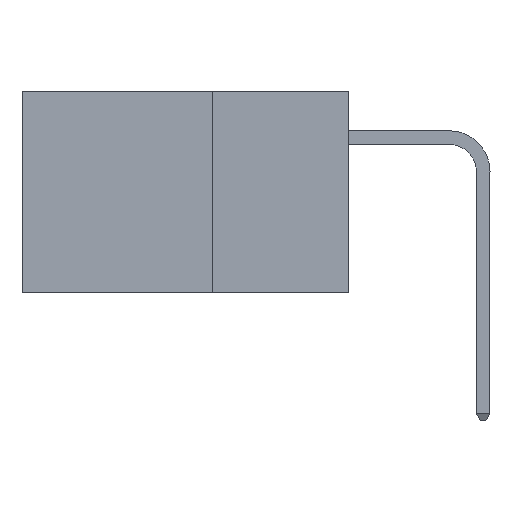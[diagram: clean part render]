
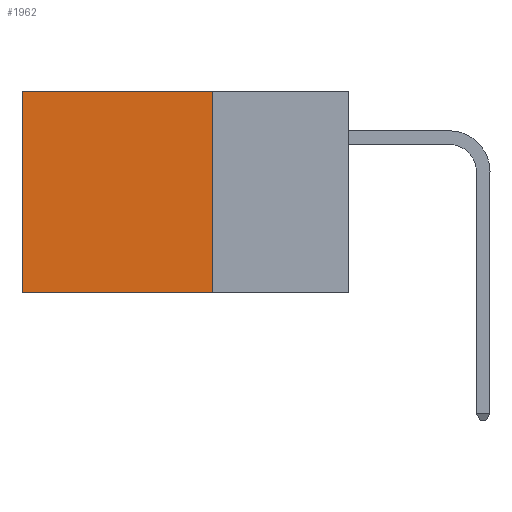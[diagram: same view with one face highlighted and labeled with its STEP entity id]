
A CAD part, left-side view. The second image highlights one B-rep face of the part: STEP entity #1962.
In plain terms, the highlighted planar face has unit normal (-1, 0, 0).
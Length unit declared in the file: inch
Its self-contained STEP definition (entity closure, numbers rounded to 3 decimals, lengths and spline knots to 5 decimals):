
#24 = CARTESIAN_POINT ( 'NONE',  ( 0.2875, 0.25, 0. ) ) ;
#293 = DIRECTION ( 'NONE',  ( 1., 0., 0. ) ) ;
#1059 = LINE ( 'NONE', #8165, #19198 ) ;
#1251 = EDGE_CURVE ( 'NONE', #1690, #9260, #20037, .T. ) ;
#1690 = VERTEX_POINT ( 'NONE', #2579 ) ;
#1962 = ADVANCED_FACE ( 'NONE', ( #7868 ), #17013, .F. ) ;
#2579 = CARTESIAN_POINT ( 'NONE',  ( 0.2875, 0.6, 0. ) ) ;
#2707 = LINE ( 'NONE', #24, #11106 ) ;
#3707 = CARTESIAN_POINT ( 'NONE',  ( 0.2875, 0.25, 0. ) ) ;
#4359 = CARTESIAN_POINT ( 'NONE',  ( 0.2875, 0.25, 0. ) ) ;
#4693 = AXIS2_PLACEMENT_3D ( 'NONE', #3707, #293, #10181 ) ;
#5417 = EDGE_LOOP ( 'NONE', ( #8640, #18408, #6620, #10983 ) ) ;
#6459 = DIRECTION ( 'NONE',  ( 0., 1., 0. ) ) ;
#6620 = ORIENTED_EDGE ( 'NONE', *, *, #13520, .F. ) ;
#6796 = DIRECTION ( 'NONE',  ( 0., 0., -1. ) ) ;
#7310 = VECTOR ( 'NONE', #19511, 39.37008 ) ;
#7457 = CARTESIAN_POINT ( 'NONE',  ( 0.2875, 0.25, 0. ) ) ;
#7610 = CARTESIAN_POINT ( 'NONE',  ( 0.2875, 0.6, 0. ) ) ;
#7868 = FACE_OUTER_BOUND ( 'NONE', #5417, .T. ) ;
#8165 = CARTESIAN_POINT ( 'NONE',  ( 0.2875, 0.25, -0.37 ) ) ;
#8640 = ORIENTED_EDGE ( 'NONE', *, *, #1251, .T. ) ;
#9008 = DIRECTION ( 'NONE',  ( 0., 0., -1. ) ) ;
#9260 = VERTEX_POINT ( 'NONE', #16653 ) ;
#10181 = DIRECTION ( 'NONE',  ( 0., 0., -1. ) ) ;
#10549 = VECTOR ( 'NONE', #9008, 39.37008 ) ;
#10983 = ORIENTED_EDGE ( 'NONE', *, *, #16628, .T. ) ;
#11106 = VECTOR ( 'NONE', #6796, 39.37008 ) ;
#13520 = EDGE_CURVE ( 'NONE', #15442, #21490, #2707, .T. ) ;
#15442 = VERTEX_POINT ( 'NONE', #7457 ) ;
#16628 = EDGE_CURVE ( 'NONE', #15442, #1690, #17072, .T. ) ;
#16653 = CARTESIAN_POINT ( 'NONE',  ( 0.2875, 0.6, -0.37 ) ) ;
#17013 = PLANE ( 'NONE',  #4693 ) ;
#17072 = LINE ( 'NONE', #4359, #7310 ) ;
#18408 = ORIENTED_EDGE ( 'NONE', *, *, #20545, .F. ) ;
#19198 = VECTOR ( 'NONE', #6459, 39.37008 ) ;
#19511 = DIRECTION ( 'NONE',  ( 0., 1., 0. ) ) ;
#20037 = LINE ( 'NONE', #7610, #10549 ) ;
#20545 = EDGE_CURVE ( 'NONE', #21490, #9260, #1059, .T. ) ;
#20939 = CARTESIAN_POINT ( 'NONE',  ( 0.2875, 0.25, -0.37 ) ) ;
#21490 = VERTEX_POINT ( 'NONE', #20939 ) ;
